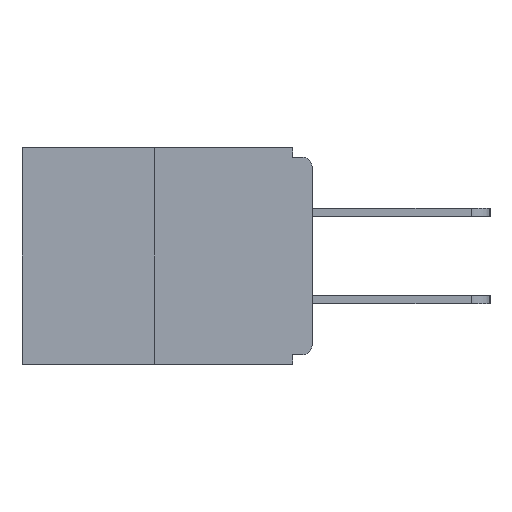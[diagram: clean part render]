
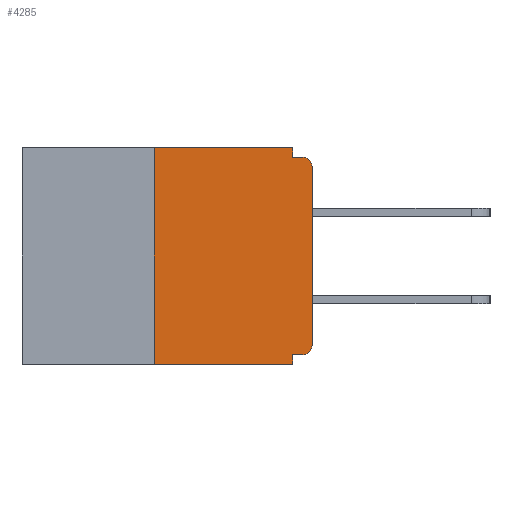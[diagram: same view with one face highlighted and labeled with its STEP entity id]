
A CAD part, left-side view. The second image highlights one B-rep face of the part: STEP entity #4285.
In plain terms, the highlighted planar face has unit normal (-1, 0, 0).
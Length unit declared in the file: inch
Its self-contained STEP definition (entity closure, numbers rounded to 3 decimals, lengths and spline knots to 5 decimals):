
#317 = EDGE_CURVE ( 'NONE', #19110, #16334, #19300, .T. ) ;
#337 = CARTESIAN_POINT ( 'NONE',  ( 0., 0.25, 0. ) ) ;
#361 = LINE ( 'NONE', #3671, #14707 ) ;
#409 = CARTESIAN_POINT ( 'NONE',  ( 0., 0., -0.03 ) ) ;
#711 = VERTEX_POINT ( 'NONE', #14394 ) ;
#832 = CARTESIAN_POINT ( 'NONE',  ( 0., 0.031, -0.343 ) ) ;
#909 = CARTESIAN_POINT ( 'NONE',  ( 0., 0.46, 0. ) ) ;
#955 = VECTOR ( 'NONE', #10586, 39.37008 ) ;
#1101 = DIRECTION ( 'NONE',  ( 0., -1., 0. ) ) ;
#1270 = EDGE_CURVE ( 'NONE', #3825, #18131, #9515, .T. ) ;
#1386 = CARTESIAN_POINT ( 'NONE',  ( 0., 0.25, -0.343 ) ) ;
#1691 = EDGE_CURVE ( 'NONE', #12490, #711, #4491, .T. ) ;
#1982 = CARTESIAN_POINT ( 'NONE',  ( 0., 0.015, -0.03 ) ) ;
#2232 = CIRCLE ( 'NONE', #5062, 0.015 ) ;
#2386 = EDGE_CURVE ( 'NONE', #16811, #19740, #361, .T. ) ;
#2394 = AXIS2_PLACEMENT_3D ( 'NONE', #11334, #14653, #2792 ) ;
#2401 = CARTESIAN_POINT ( 'NONE',  ( 0., 0.46, -0.343 ) ) ;
#2427 = LINE ( 'NONE', #10525, #10690 ) ;
#2674 = CARTESIAN_POINT ( 'NONE',  ( 0., 0.031, -0.328 ) ) ;
#2792 = DIRECTION ( 'NONE',  ( 0., 0., -1. ) ) ;
#3119 = CARTESIAN_POINT ( 'NONE',  ( 0., 0., -0.313 ) ) ;
#3187 = EDGE_CURVE ( 'NONE', #12490, #19110, #17016, .T. ) ;
#3477 = ORIENTED_EDGE ( 'NONE', *, *, #3187, .F. ) ;
#3671 = CARTESIAN_POINT ( 'NONE',  ( 0., 0., -0.328 ) ) ;
#3767 = DIRECTION ( 'NONE',  ( 0., 0., -1. ) ) ;
#3823 = CARTESIAN_POINT ( 'NONE',  ( 0., 0.25, 0. ) ) ;
#3825 = VERTEX_POINT ( 'NONE', #8021 ) ;
#4061 = DIRECTION ( 'NONE',  ( 0., -1., 0. ) ) ;
#4092 = DIRECTION ( 'NONE',  ( 0., 0., 1. ) ) ;
#4267 = VERTEX_POINT ( 'NONE', #3119 ) ;
#4285 = ADVANCED_FACE ( 'NONE', ( #13206 ), #9880, .F. ) ;
#4435 = ORIENTED_EDGE ( 'NONE', *, *, #1270, .F. ) ;
#4491 = LINE ( 'NONE', #2401, #11385 ) ;
#4518 = ORIENTED_EDGE ( 'NONE', *, *, #21286, .F. ) ;
#4970 = EDGE_CURVE ( 'NONE', #4267, #16588, #2427, .T. ) ;
#5062 = AXIS2_PLACEMENT_3D ( 'NONE', #15339, #14211, #10466 ) ;
#5500 = VECTOR ( 'NONE', #1101, 39.37008 ) ;
#5754 = CARTESIAN_POINT ( 'NONE',  ( 0., 0.031, 0. ) ) ;
#6101 = EDGE_CURVE ( 'NONE', #16588, #18131, #21692, .T. ) ;
#6799 = CARTESIAN_POINT ( 'NONE',  ( 0., 0.015, -0.328 ) ) ;
#7066 = DIRECTION ( 'NONE',  ( -1., 0., 0. ) ) ;
#7084 = LINE ( 'NONE', #5754, #17602 ) ;
#7214 = DIRECTION ( 'NONE',  ( 0., 1., 0. ) ) ;
#7871 = EDGE_CURVE ( 'NONE', #16811, #4267, #2232, .T. ) ;
#8021 = CARTESIAN_POINT ( 'NONE',  ( 0., 0.031, -0.015 ) ) ;
#9140 = LINE ( 'NONE', #832, #17796 ) ;
#9202 = DIRECTION ( 'NONE',  ( 0., -1., 0. ) ) ;
#9515 = LINE ( 'NONE', #16275, #5500 ) ;
#9880 = PLANE ( 'NONE',  #2394 ) ;
#10466 = DIRECTION ( 'NONE',  ( 0., 0., -1. ) ) ;
#10525 = CARTESIAN_POINT ( 'NONE',  ( 0., 0., 0. ) ) ;
#10586 = DIRECTION ( 'NONE',  ( 0., 0., 1. ) ) ;
#10681 = ORIENTED_EDGE ( 'NONE', *, *, #2386, .F. ) ;
#10690 = VECTOR ( 'NONE', #4092, 39.37008 ) ;
#11334 = CARTESIAN_POINT ( 'NONE',  ( 0., 0.46, 0. ) ) ;
#11385 = VECTOR ( 'NONE', #4061, 39.37008 ) ;
#12224 = ORIENTED_EDGE ( 'NONE', *, *, #7871, .T. ) ;
#12490 = VERTEX_POINT ( 'NONE', #1386 ) ;
#12575 = ORIENTED_EDGE ( 'NONE', *, *, #6101, .T. ) ;
#12820 = ORIENTED_EDGE ( 'NONE', *, *, #15912, .F. ) ;
#13206 = FACE_OUTER_BOUND ( 'NONE', #19036, .T. ) ;
#13612 = ORIENTED_EDGE ( 'NONE', *, *, #317, .F. ) ;
#13835 = DIRECTION ( 'NONE',  ( 0., 0., -1. ) ) ;
#14118 = ORIENTED_EDGE ( 'NONE', *, *, #4970, .T. ) ;
#14211 = DIRECTION ( 'NONE',  ( -1., 0., 0. ) ) ;
#14394 = CARTESIAN_POINT ( 'NONE',  ( 0., 0.031, -0.343 ) ) ;
#14653 = DIRECTION ( 'NONE',  ( 1., 0., 0. ) ) ;
#14707 = VECTOR ( 'NONE', #7214, 39.37008 ) ;
#15339 = CARTESIAN_POINT ( 'NONE',  ( 0., 0.015, -0.313 ) ) ;
#15388 = ORIENTED_EDGE ( 'NONE', *, *, #1691, .T. ) ;
#15898 = DIRECTION ( 'NONE',  ( 0., 0., -1. ) ) ;
#15912 = EDGE_CURVE ( 'NONE', #19740, #711, #9140, .T. ) ;
#16275 = CARTESIAN_POINT ( 'NONE',  ( 0., 0., -0.015 ) ) ;
#16334 = VERTEX_POINT ( 'NONE', #21256 ) ;
#16588 = VERTEX_POINT ( 'NONE', #409 ) ;
#16811 = VERTEX_POINT ( 'NONE', #6799 ) ;
#17016 = LINE ( 'NONE', #3823, #955 ) ;
#17602 = VECTOR ( 'NONE', #3767, 39.37008 ) ;
#17796 = VECTOR ( 'NONE', #15898, 39.37008 ) ;
#18131 = VERTEX_POINT ( 'NONE', #21661 ) ;
#18498 = AXIS2_PLACEMENT_3D ( 'NONE', #1982, #7066, #13835 ) ;
#19036 = EDGE_LOOP ( 'NONE', ( #13612, #3477, #15388, #12820, #10681, #12224, #14118, #12575, #4435, #4518 ) ) ;
#19110 = VERTEX_POINT ( 'NONE', #337 ) ;
#19300 = LINE ( 'NONE', #909, #20638 ) ;
#19740 = VERTEX_POINT ( 'NONE', #2674 ) ;
#20638 = VECTOR ( 'NONE', #9202, 39.37008 ) ;
#21256 = CARTESIAN_POINT ( 'NONE',  ( 0., 0.031, 0. ) ) ;
#21286 = EDGE_CURVE ( 'NONE', #16334, #3825, #7084, .T. ) ;
#21661 = CARTESIAN_POINT ( 'NONE',  ( 0., 0.015, -0.015 ) ) ;
#21692 = CIRCLE ( 'NONE', #18498, 0.015 ) ;
